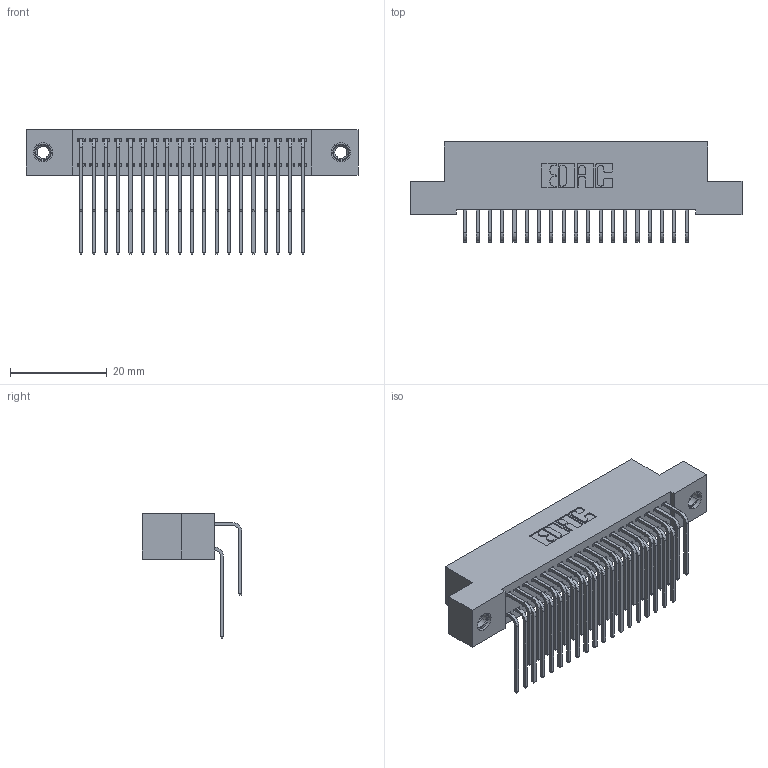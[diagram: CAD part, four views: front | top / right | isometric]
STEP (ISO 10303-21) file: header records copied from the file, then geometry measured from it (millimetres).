
FILE_DESCRIPTION (( 'STEP AP203' ), '1' );
FILE_NAME ('392-038-559-207.STEP', '2018-08-16T06:04:14', ( '' ), ( '' ), 'SwSTEP 2.0', 'SolidWorks 2016', '' );
FILE_SCHEMA (( 'CONFIG_CONTROL_DESIGN' ));
Length unit declared in the file: inch
Products named in the file (5): 342 Part_TI; 345-292-001_558 559 Tail - 1; 345-292-001_559 Tail - 2; 345-250-001_345-250-005-103; 392-038-559-207
Assembly tree (41 placements, depth 2):
  392-038-559-207
    342 Part_TI
    345-292-001_558 559 Tail - 1  x19
    345-292-001_559 Tail - 2  x19
    345-250-001_345-250-005-103  x2
Bounding box: 68.58 x 20.64 x 25.78 mm (x, y, z)
Volume: 6259.6 mm3; surface area: 10639.7 mm2
Topology: 41 solids, 41 shells, 2222 faces, 6553 edges, 4310 vertices
Faces by surface type: plane 1542, cylinder 664, cone 12, torus 4
Entity records: 18036 total; most frequent: CARTESIAN_POINT 3048, ORIENTED_EDGE 2926, DIRECTION 2657, EDGE_CURVE 1463, VECTOR 1275, LINE 1275, VERTEX_POINT 968, AXIS2_PLACEMENT_3D 691
